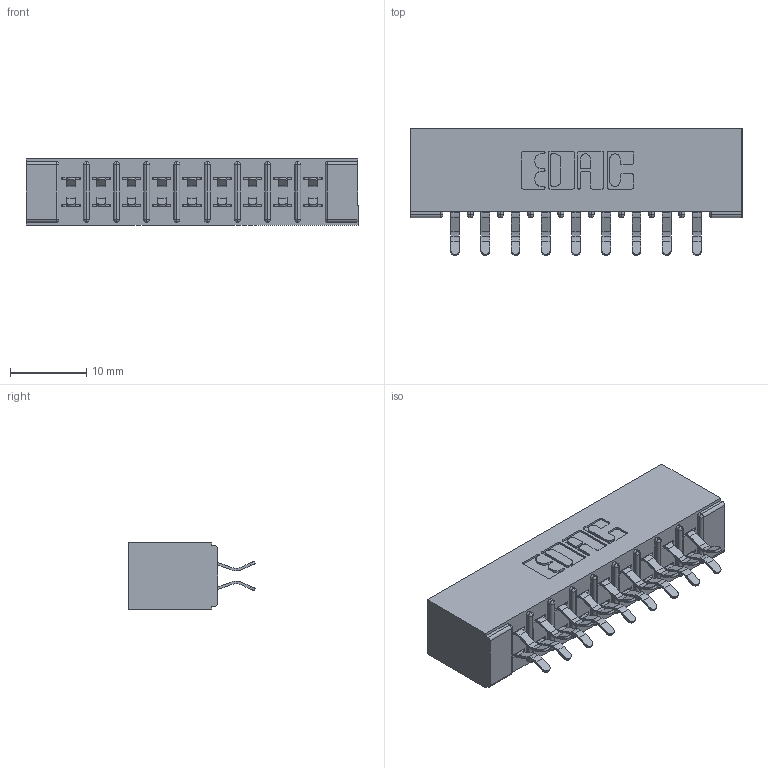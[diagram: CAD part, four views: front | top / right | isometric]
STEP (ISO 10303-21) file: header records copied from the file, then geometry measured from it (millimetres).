
FILE_DESCRIPTION (( 'STEP AP203' ), '1' );
FILE_NAME ('355-018-556-201.STEP', '2019-09-11T02:56:19', ( '' ), ( '' ), 'SwSTEP 2.0', 'SolidWorks 2016', '' );
FILE_SCHEMA (( 'CONFIG_CONTROL_DESIGN' ));
Length unit declared in the file: inch
Products named in the file (3): 305-290-001_556; 355-018-556-201; 305 Part_No Mounting
Assembly tree (19 placements, depth 2):
  355-018-556-201
    305 Part_No Mounting
    305-290-001_556  x18
Bounding box: 43.54 x 16.64 x 8.71 mm (x, y, z)
Volume: 2934.2 mm3; surface area: 5358.8 mm2
Topology: 19 solids, 19 shells, 1116 faces, 3199 edges, 2082 vertices
Faces by surface type: plane 622, cylinder 458, sphere 36
Entity records: 13706 total; most frequent: CARTESIAN_POINT 2269, ORIENTED_EDGE 2246, DIRECTION 2223, EDGE_CURVE 1123, LINE 871, VECTOR 871, VERTEX_POINT 722, AXIS2_PLACEMENT_3D 676
